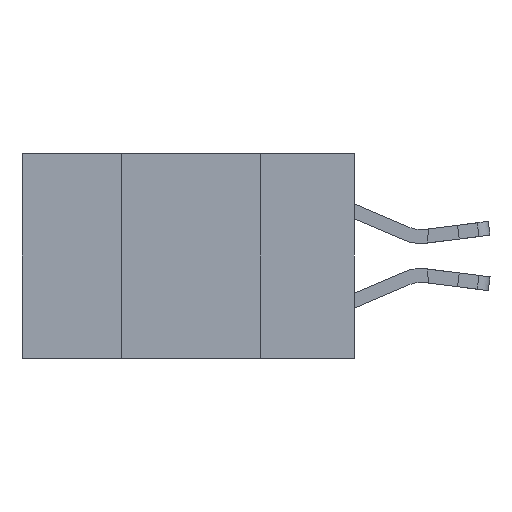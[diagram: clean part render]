
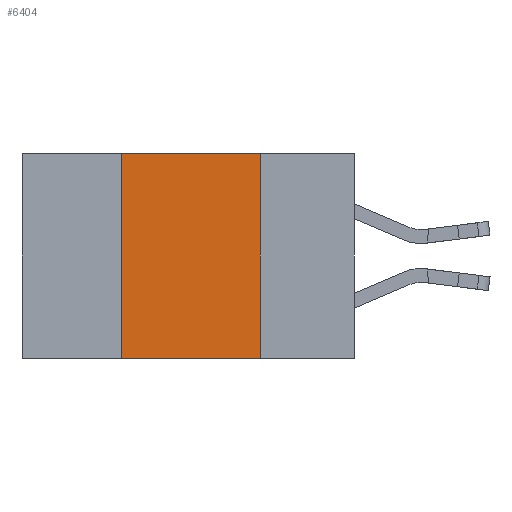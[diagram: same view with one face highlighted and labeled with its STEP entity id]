
A CAD part, left-side view. The second image highlights one B-rep face of the part: STEP entity #6404.
In plain terms, the highlighted planar face has unit normal (-1, 0, 0).
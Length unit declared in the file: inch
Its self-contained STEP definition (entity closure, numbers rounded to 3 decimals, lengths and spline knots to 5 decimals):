
#42 = VERTEX_POINT ( 'NONE', #2732 ) ;
#1708 = VECTOR ( 'NONE', #11693, 39.37008 ) ;
#2090 = CARTESIAN_POINT ( 'NONE',  ( 0., 0.42, 0. ) ) ;
#2672 = VECTOR ( 'NONE', #5471, 39.37008 ) ;
#2732 = CARTESIAN_POINT ( 'NONE',  ( 0., 0.17, 0. ) ) ;
#3233 = CARTESIAN_POINT ( 'NONE',  ( 0., 0.6, -0.37 ) ) ;
#3433 = LINE ( 'NONE', #3233, #1708 ) ;
#3873 = VECTOR ( 'NONE', #14434, 39.37008 ) ;
#4482 = VERTEX_POINT ( 'NONE', #16224 ) ;
#5405 = DIRECTION ( 'NONE',  ( 1., 0., 0. ) ) ;
#5471 = DIRECTION ( 'NONE',  ( 0., 0., -1. ) ) ;
#6404 = ADVANCED_FACE ( 'NONE', ( #8159 ), #11198, .F. ) ;
#6419 = EDGE_CURVE ( 'NONE', #42, #7924, #17545, .T. ) ;
#6560 = LINE ( 'NONE', #13090, #3873 ) ;
#6816 = CARTESIAN_POINT ( 'NONE',  ( 0., 0.17, 0. ) ) ;
#7275 = EDGE_CURVE ( 'NONE', #8084, #42, #14667, .T. ) ;
#7924 = VERTEX_POINT ( 'NONE', #17580 ) ;
#8084 = VERTEX_POINT ( 'NONE', #2090 ) ;
#8159 = FACE_OUTER_BOUND ( 'NONE', #9387, .T. ) ;
#8279 = DIRECTION ( 'NONE',  ( 0., 0., -1. ) ) ;
#9387 = EDGE_LOOP ( 'NONE', ( #14167, #10328, #12097, #16379 ) ) ;
#10328 = ORIENTED_EDGE ( 'NONE', *, *, #7275, .F. ) ;
#10887 = EDGE_CURVE ( 'NONE', #4482, #8084, #6560, .T. ) ;
#11198 = PLANE ( 'NONE',  #12907 ) ;
#11693 = DIRECTION ( 'NONE',  ( 0., -1., 0. ) ) ;
#12097 = ORIENTED_EDGE ( 'NONE', *, *, #10887, .F. ) ;
#12907 = AXIS2_PLACEMENT_3D ( 'NONE', #16614, #5405, #8279 ) ;
#12927 = DIRECTION ( 'NONE',  ( 0., -1., 0. ) ) ;
#13090 = CARTESIAN_POINT ( 'NONE',  ( 0., 0.42, 0. ) ) ;
#14167 = ORIENTED_EDGE ( 'NONE', *, *, #6419, .F. ) ;
#14434 = DIRECTION ( 'NONE',  ( 0., 0., 1. ) ) ;
#14667 = LINE ( 'NONE', #15747, #15085 ) ;
#14678 = EDGE_CURVE ( 'NONE', #4482, #7924, #3433, .T. ) ;
#15085 = VECTOR ( 'NONE', #12927, 39.37008 ) ;
#15747 = CARTESIAN_POINT ( 'NONE',  ( 0., 0.6, 0. ) ) ;
#16224 = CARTESIAN_POINT ( 'NONE',  ( 0., 0.42, -0.37 ) ) ;
#16379 = ORIENTED_EDGE ( 'NONE', *, *, #14678, .T. ) ;
#16614 = CARTESIAN_POINT ( 'NONE',  ( 0., 0.6, 0. ) ) ;
#17545 = LINE ( 'NONE', #6816, #2672 ) ;
#17580 = CARTESIAN_POINT ( 'NONE',  ( 0., 0.17, -0.37 ) ) ;
